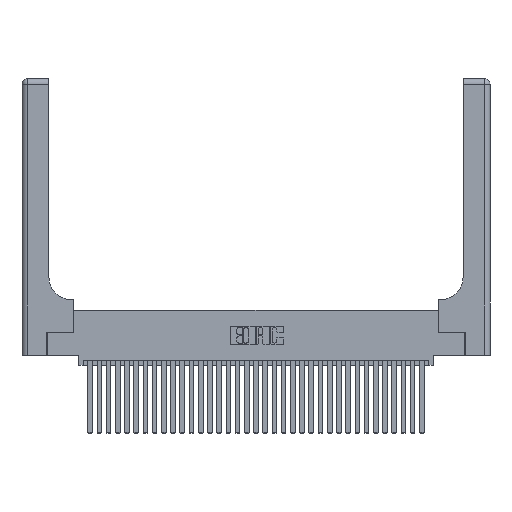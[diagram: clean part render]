
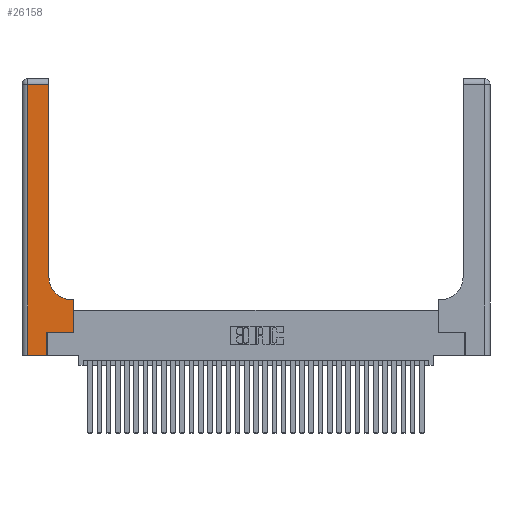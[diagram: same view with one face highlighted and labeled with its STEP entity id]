
A CAD part, top view. The second image highlights one B-rep face of the part: STEP entity #26158.
In plain terms, the highlighted planar face has unit normal (0, 0, 1).
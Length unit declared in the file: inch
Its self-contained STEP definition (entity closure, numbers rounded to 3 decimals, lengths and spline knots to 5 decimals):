
#177 = DIRECTION ( 'NONE',  ( -1., 0., 0. ) ) ;
#523 = VERTEX_POINT ( 'NONE', #30878 ) ;
#1174 = VECTOR ( 'NONE', #22385, 39.37008 ) ;
#1992 = CARTESIAN_POINT ( 'NONE',  ( 0.269, 0.25, 0.37 ) ) ;
#2256 = LINE ( 'NONE', #28011, #17339 ) ;
#2361 = CARTESIAN_POINT ( 'NONE',  ( 0.269, 0., 0.37 ) ) ;
#2547 = LINE ( 'NONE', #28160, #1174 ) ;
#2580 = EDGE_CURVE ( 'NONE', #523, #12517, #14980, .T. ) ;
#2610 = VERTEX_POINT ( 'NONE', #1992 ) ;
#2689 = DIRECTION ( 'NONE',  ( 0., 1., 0. ) ) ;
#2844 = CARTESIAN_POINT ( 'NONE',  ( 0., 3., 0.37 ) ) ;
#2934 = LINE ( 'NONE', #2361, #7989 ) ;
#3807 = ORIENTED_EDGE ( 'NONE', *, *, #17991, .T. ) ;
#3926 = LINE ( 'NONE', #18244, #7332 ) ;
#5395 = ORIENTED_EDGE ( 'NONE', *, *, #2580, .T. ) ;
#5717 = DIRECTION ( 'NONE',  ( 0., 0., -1. ) ) ;
#5740 = VERTEX_POINT ( 'NONE', #15804 ) ;
#6111 = DIRECTION ( 'NONE',  ( -1., 0., 0. ) ) ;
#6577 = AXIS2_PLACEMENT_3D ( 'NONE', #16495, #5717, #8409 ) ;
#7332 = VECTOR ( 'NONE', #9784, 39.37008 ) ;
#7989 = VECTOR ( 'NONE', #2689, 39.37008 ) ;
#8273 = VECTOR ( 'NONE', #22127, 39.37008 ) ;
#8409 = DIRECTION ( 'NONE',  ( 1., 0., 0. ) ) ;
#9587 = ORIENTED_EDGE ( 'NONE', *, *, #10400, .T. ) ;
#9784 = DIRECTION ( 'NONE',  ( 1., 0., 0. ) ) ;
#10315 = EDGE_CURVE ( 'NONE', #29390, #18015, #21952, .T. ) ;
#10400 = EDGE_CURVE ( 'NONE', #21368, #523, #17316, .T. ) ;
#11296 = AXIS2_PLACEMENT_3D ( 'NONE', #2844, #13714, #177 ) ;
#11350 = VECTOR ( 'NONE', #26938, 39.37008 ) ;
#11596 = CARTESIAN_POINT ( 'NONE',  ( 0.2915, 0.6, 0.37 ) ) ;
#11889 = FACE_OUTER_BOUND ( 'NONE', #31655, .T. ) ;
#11904 = DIRECTION ( 'NONE',  ( 0., -1., 0. ) ) ;
#12517 = VERTEX_POINT ( 'NONE', #28676 ) ;
#13507 = PLANE ( 'NONE',  #11296 ) ;
#13714 = DIRECTION ( 'NONE',  ( 0., 0., -1. ) ) ;
#13904 = VERTEX_POINT ( 'NONE', #21546 ) ;
#13991 = VERTEX_POINT ( 'NONE', #19838 ) ;
#14980 = LINE ( 'NONE', #33836, #8273 ) ;
#15260 = CARTESIAN_POINT ( 'NONE',  ( 0.2915, 3., 0.37 ) ) ;
#15804 = CARTESIAN_POINT ( 'NONE',  ( 0.5585, 0.25, 0.37 ) ) ;
#16495 = CARTESIAN_POINT ( 'NONE',  ( 0.5415, 0.85, 0.37 ) ) ;
#17088 = ORIENTED_EDGE ( 'NONE', *, *, #26679, .T. ) ;
#17316 = LINE ( 'NONE', #15260, #32069 ) ;
#17339 = VECTOR ( 'NONE', #11904, 39.37008 ) ;
#17991 = EDGE_CURVE ( 'NONE', #12517, #13904, #2256, .T. ) ;
#18015 = VERTEX_POINT ( 'NONE', #19544 ) ;
#18244 = CARTESIAN_POINT ( 'NONE',  ( 0.269, 0.25, 0.37 ) ) ;
#18253 = ORIENTED_EDGE ( 'NONE', *, *, #28641, .T. ) ;
#18321 = ORIENTED_EDGE ( 'NONE', *, *, #25864, .T. ) ;
#19045 = ORIENTED_EDGE ( 'NONE', *, *, #19074, .T. ) ;
#19074 = EDGE_CURVE ( 'NONE', #5740, #29390, #2547, .T. ) ;
#19544 = CARTESIAN_POINT ( 'NONE',  ( 0.5415, 0.6, 0.37 ) ) ;
#19838 = CARTESIAN_POINT ( 'NONE',  ( 0.269, 0., 0.37 ) ) ;
#21368 = VERTEX_POINT ( 'NONE', #23465 ) ;
#21546 = CARTESIAN_POINT ( 'NONE',  ( 0.06, 0., 0.37 ) ) ;
#21952 = LINE ( 'NONE', #11596, #32879 ) ;
#22127 = DIRECTION ( 'NONE',  ( -1., 0., 0. ) ) ;
#22281 = LINE ( 'NONE', #29986, #11350 ) ;
#22385 = DIRECTION ( 'NONE',  ( 0., 1., 0. ) ) ;
#23465 = CARTESIAN_POINT ( 'NONE',  ( 0.2915, 0.85, 0.37 ) ) ;
#25072 = CARTESIAN_POINT ( 'NONE',  ( 0.5585, 0.6, 0.37 ) ) ;
#25864 = EDGE_CURVE ( 'NONE', #2610, #5740, #3926, .T. ) ;
#26158 = ADVANCED_FACE ( 'NONE', ( #11889 ), #13507, .F. ) ;
#26679 = EDGE_CURVE ( 'NONE', #18015, #21368, #34206, .T. ) ;
#26938 = DIRECTION ( 'NONE',  ( 1., 0., 0. ) ) ;
#27089 = ORIENTED_EDGE ( 'NONE', *, *, #27800, .T. ) ;
#27800 = EDGE_CURVE ( 'NONE', #13904, #13991, #22281, .T. ) ;
#28011 = CARTESIAN_POINT ( 'NONE',  ( 0.06, 3., 0.37 ) ) ;
#28160 = CARTESIAN_POINT ( 'NONE',  ( 0.5585, 0.25, 0.37 ) ) ;
#28641 = EDGE_CURVE ( 'NONE', #13991, #2610, #2934, .T. ) ;
#28676 = CARTESIAN_POINT ( 'NONE',  ( 0.06, 2.94, 0.37 ) ) ;
#29390 = VERTEX_POINT ( 'NONE', #25072 ) ;
#29956 = DIRECTION ( 'NONE',  ( 0., 1., 0. ) ) ;
#29986 = CARTESIAN_POINT ( 'NONE',  ( 0., 0., 0.37 ) ) ;
#30878 = CARTESIAN_POINT ( 'NONE',  ( 0.2915, 2.94, 0.37 ) ) ;
#31349 = ORIENTED_EDGE ( 'NONE', *, *, #10315, .T. ) ;
#31655 = EDGE_LOOP ( 'NONE', ( #9587, #5395, #3807, #27089, #18253, #18321, #19045, #31349, #17088 ) ) ;
#32069 = VECTOR ( 'NONE', #29956, 39.37008 ) ;
#32879 = VECTOR ( 'NONE', #6111, 39.37008 ) ;
#33836 = CARTESIAN_POINT ( 'NONE',  ( 0., 2.94, 0.37 ) ) ;
#34206 = CIRCLE ( 'NONE', #6577, 0.25 ) ;
